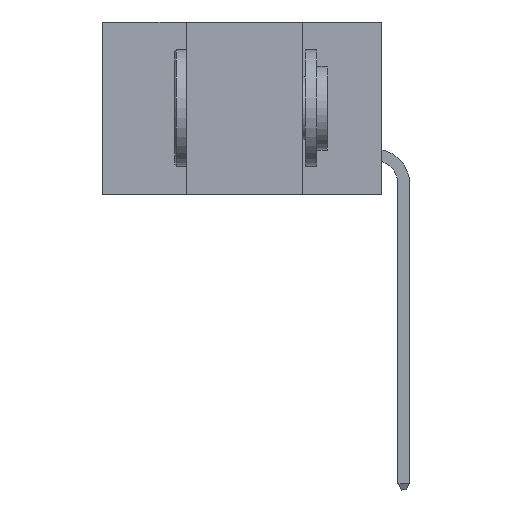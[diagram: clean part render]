
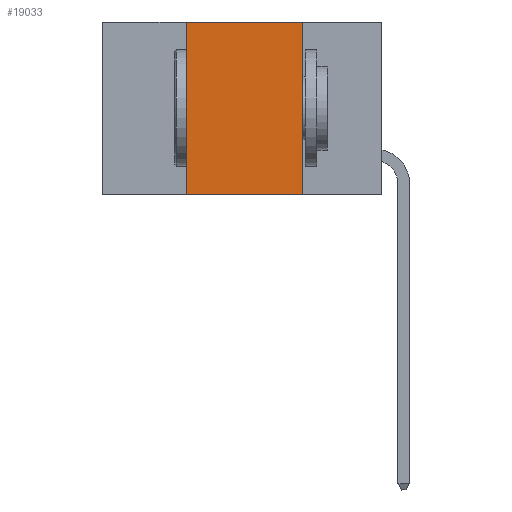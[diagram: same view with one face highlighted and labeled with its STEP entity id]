
A CAD part, left-side view. The second image highlights one B-rep face of the part: STEP entity #19033.
In plain terms, the highlighted planar face has unit normal (-1, 0, 0).
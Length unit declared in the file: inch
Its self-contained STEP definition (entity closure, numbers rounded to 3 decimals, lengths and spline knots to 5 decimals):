
#907 = VERTEX_POINT ( 'NONE', #5077 ) ;
#1834 = DIRECTION ( 'NONE',  ( 0., 0., -1. ) ) ;
#3746 = CARTESIAN_POINT ( 'NONE',  ( 0., 0.17, 0. ) ) ;
#4430 = DIRECTION ( 'NONE',  ( 0., 0., -1. ) ) ;
#4700 = LINE ( 'NONE', #3746, #16430 ) ;
#5077 = CARTESIAN_POINT ( 'NONE',  ( 0., 0.17, -0.37 ) ) ;
#5749 = VECTOR ( 'NONE', #28570, 39.37008 ) ;
#5875 = CARTESIAN_POINT ( 'NONE',  ( 0., 0.42, 0. ) ) ;
#5884 = VERTEX_POINT ( 'NONE', #27474 ) ;
#6961 = VERTEX_POINT ( 'NONE', #23672 ) ;
#6973 = ORIENTED_EDGE ( 'NONE', *, *, #17383, .F. ) ;
#7328 = DIRECTION ( 'NONE',  ( 0., -1., 0. ) ) ;
#10702 = LINE ( 'NONE', #5875, #5749 ) ;
#11019 = ORIENTED_EDGE ( 'NONE', *, *, #17993, .F. ) ;
#15292 = ORIENTED_EDGE ( 'NONE', *, *, #24896, .F. ) ;
#15766 = PLANE ( 'NONE',  #25229 ) ;
#15953 = DIRECTION ( 'NONE',  ( 1., 0., 0. ) ) ;
#16182 = VERTEX_POINT ( 'NONE', #24345 ) ;
#16430 = VECTOR ( 'NONE', #1834, 39.37008 ) ;
#16769 = EDGE_LOOP ( 'NONE', ( #6973, #15292, #11019, #24216 ) ) ;
#17383 = EDGE_CURVE ( 'NONE', #6961, #907, #4700, .T. ) ;
#17993 = EDGE_CURVE ( 'NONE', #16182, #5884, #10702, .T. ) ;
#19033 = ADVANCED_FACE ( 'NONE', ( #24148 ), #15766, .F. ) ;
#19439 = LINE ( 'NONE', #27082, #24035 ) ;
#20836 = EDGE_CURVE ( 'NONE', #16182, #907, #19439, .T. ) ;
#22753 = DIRECTION ( 'NONE',  ( 0., -1., 0. ) ) ;
#23203 = CARTESIAN_POINT ( 'NONE',  ( 0., 0.6, 0. ) ) ;
#23619 = LINE ( 'NONE', #23203, #26054 ) ;
#23672 = CARTESIAN_POINT ( 'NONE',  ( 0., 0.17, 0. ) ) ;
#24035 = VECTOR ( 'NONE', #22753, 39.37008 ) ;
#24148 = FACE_OUTER_BOUND ( 'NONE', #16769, .T. ) ;
#24216 = ORIENTED_EDGE ( 'NONE', *, *, #20836, .T. ) ;
#24345 = CARTESIAN_POINT ( 'NONE',  ( 0., 0.42, -0.37 ) ) ;
#24896 = EDGE_CURVE ( 'NONE', #5884, #6961, #23619, .T. ) ;
#25229 = AXIS2_PLACEMENT_3D ( 'NONE', #26094, #15953, #4430 ) ;
#26054 = VECTOR ( 'NONE', #7328, 39.37008 ) ;
#26094 = CARTESIAN_POINT ( 'NONE',  ( 0., 0.6, 0. ) ) ;
#27082 = CARTESIAN_POINT ( 'NONE',  ( 0., 0.6, -0.37 ) ) ;
#27474 = CARTESIAN_POINT ( 'NONE',  ( 0., 0.42, 0. ) ) ;
#28570 = DIRECTION ( 'NONE',  ( 0., 0., 1. ) ) ;
